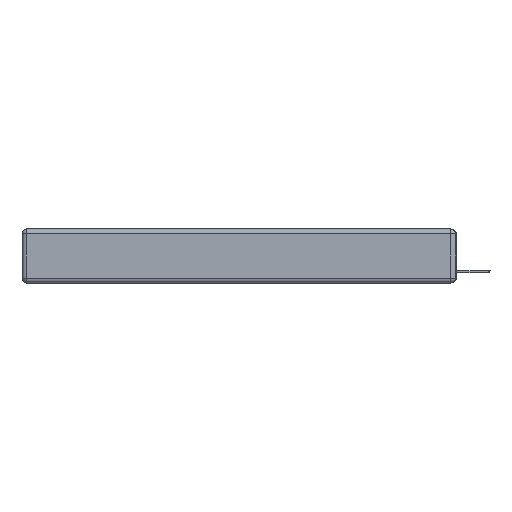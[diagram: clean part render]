
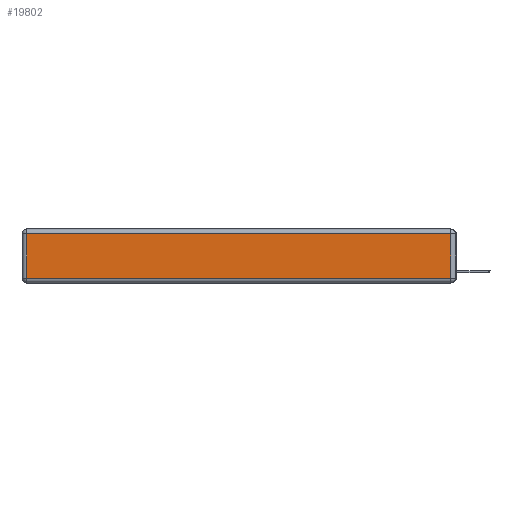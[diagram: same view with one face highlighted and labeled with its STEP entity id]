
A CAD part, left-side view. The second image highlights one B-rep face of the part: STEP entity #19802.
In plain terms, the highlighted planar face has unit normal (-1, 0, 0).
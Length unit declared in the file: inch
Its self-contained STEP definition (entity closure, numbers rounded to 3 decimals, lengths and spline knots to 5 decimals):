
#692 = PLANE ( 'NONE',  #8192 ) ;
#1861 = LINE ( 'NONE', #7604, #2157 ) ;
#2071 = ORIENTED_EDGE ( 'NONE', *, *, #6565, .T. ) ;
#2157 = VECTOR ( 'NONE', #13356, 39.37008 ) ;
#2867 = EDGE_CURVE ( 'NONE', #19278, #22214, #17608, .T. ) ;
#3081 = VERTEX_POINT ( 'NONE', #16878 ) ;
#3251 = EDGE_CURVE ( 'NONE', #22214, #16634, #20196, .T. ) ;
#3857 = CARTESIAN_POINT ( 'NONE',  ( 0., 2.72, -0.03 ) ) ;
#4503 = CARTESIAN_POINT ( 'NONE',  ( 0., 2.72, -0.313 ) ) ;
#4907 = EDGE_CURVE ( 'NONE', #3081, #19278, #23908, .T. ) ;
#6565 = EDGE_CURVE ( 'NONE', #16634, #3081, #1861, .T. ) ;
#7544 = DIRECTION ( 'NONE',  ( 0., 0., 1. ) ) ;
#7604 = CARTESIAN_POINT ( 'NONE',  ( 0., 0., -0.313 ) ) ;
#7781 = CARTESIAN_POINT ( 'NONE',  ( 0., 0.03, -0.343 ) ) ;
#8192 = AXIS2_PLACEMENT_3D ( 'NONE', #9747, #13546, #15257 ) ;
#8288 = CARTESIAN_POINT ( 'NONE',  ( 0., 2.72, -0.343 ) ) ;
#8961 = DIRECTION ( 'NONE',  ( 0., 1., 0. ) ) ;
#9207 = VECTOR ( 'NONE', #8961, 39.37008 ) ;
#9747 = CARTESIAN_POINT ( 'NONE',  ( 0., 0., -0.343 ) ) ;
#10095 = ORIENTED_EDGE ( 'NONE', *, *, #4907, .T. ) ;
#11267 = FACE_OUTER_BOUND ( 'NONE', #15354, .T. ) ;
#13356 = DIRECTION ( 'NONE',  ( 0., -1., 0. ) ) ;
#13546 = DIRECTION ( 'NONE',  ( -1., 0., 0. ) ) ;
#14693 = VECTOR ( 'NONE', #19043, 39.37008 ) ;
#15257 = DIRECTION ( 'NONE',  ( 0., 0., 1. ) ) ;
#15354 = EDGE_LOOP ( 'NONE', ( #2071, #10095, #22353, #18497 ) ) ;
#16634 = VERTEX_POINT ( 'NONE', #4503 ) ;
#16878 = CARTESIAN_POINT ( 'NONE',  ( 0., 0.03, -0.313 ) ) ;
#17608 = LINE ( 'NONE', #18103, #9207 ) ;
#18103 = CARTESIAN_POINT ( 'NONE',  ( 0., 2.75, -0.03 ) ) ;
#18497 = ORIENTED_EDGE ( 'NONE', *, *, #3251, .T. ) ;
#18936 = VECTOR ( 'NONE', #7544, 39.37008 ) ;
#19043 = DIRECTION ( 'NONE',  ( 0., 0., -1. ) ) ;
#19278 = VERTEX_POINT ( 'NONE', #22578 ) ;
#19802 = ADVANCED_FACE ( 'NONE', ( #11267 ), #692, .T. ) ;
#20196 = LINE ( 'NONE', #8288, #14693 ) ;
#22214 = VERTEX_POINT ( 'NONE', #3857 ) ;
#22353 = ORIENTED_EDGE ( 'NONE', *, *, #2867, .T. ) ;
#22578 = CARTESIAN_POINT ( 'NONE',  ( 0., 0.03, -0.03 ) ) ;
#23908 = LINE ( 'NONE', #7781, #18936 ) ;
